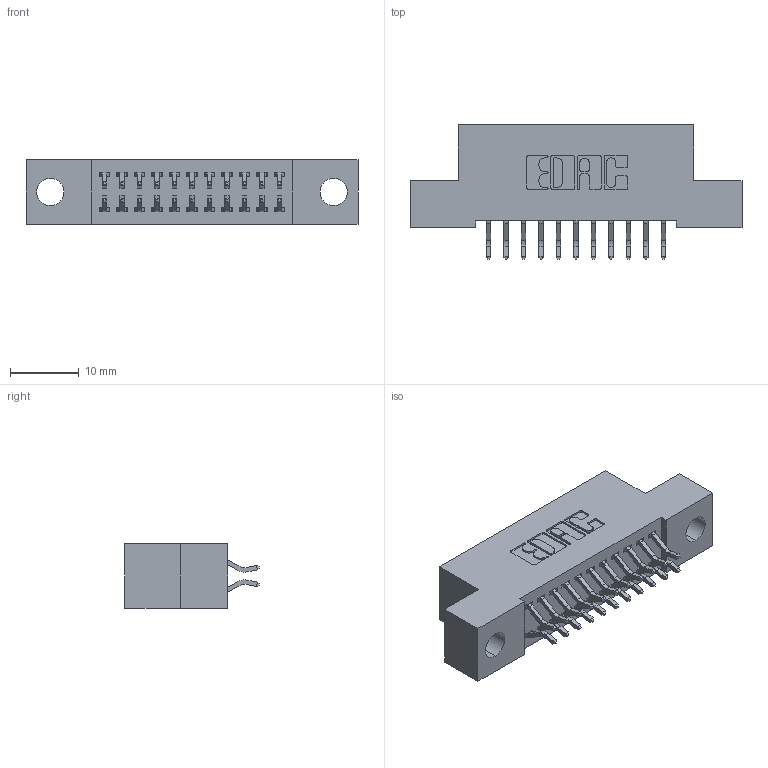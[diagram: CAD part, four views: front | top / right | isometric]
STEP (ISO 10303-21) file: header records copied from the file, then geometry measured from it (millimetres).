
FILE_DESCRIPTION (( 'STEP AP203' ), '1' );
FILE_NAME ('392-022-556-204.STEP', '2018-08-15T13:03:56', ( '' ), ( '' ), 'SwSTEP 2.0', 'SolidWorks 2016', '' );
FILE_SCHEMA (( 'CONFIG_CONTROL_DESIGN' ));
Length unit declared in the file: inch
Products named in the file (3): 342 Part_.156 TH; 345-292-001_556 Tail; 392-022-556-204
Assembly tree (23 placements, depth 2):
  392-022-556-204
    342 Part_.156 TH
    345-292-001_556 Tail  x22
Bounding box: 48.26 x 19.58 x 9.4 mm (x, y, z)
Volume: 4101.8 mm3; surface area: 5715.8 mm2
Topology: 23 solids, 23 shells, 1386 faces, 4105 edges, 2706 vertices
Faces by surface type: plane 946, cylinder 440
Entity records: 11177 total; most frequent: CARTESIAN_POINT 1902, ORIENTED_EDGE 1826, DIRECTION 1669, EDGE_CURVE 913, VECTOR 777, LINE 777, VERTEX_POINT 606, AXIS2_PLACEMENT_3D 446
